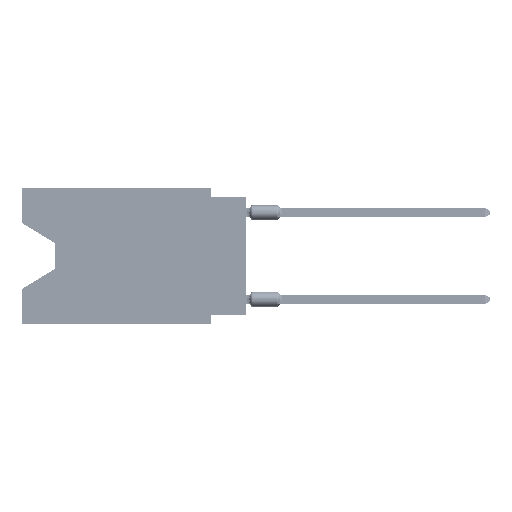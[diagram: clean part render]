
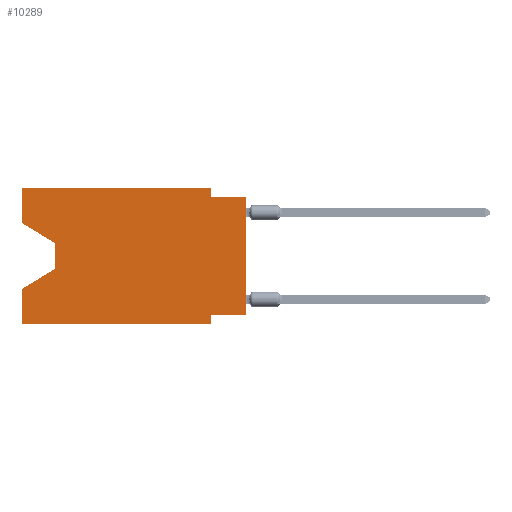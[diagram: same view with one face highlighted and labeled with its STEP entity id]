
A CAD part, left-side view. The second image highlights one B-rep face of the part: STEP entity #10289.
In plain terms, the highlighted planar face has unit normal (-1, 0, 0).
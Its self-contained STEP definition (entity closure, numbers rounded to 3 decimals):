
#3609 = DIRECTION ( 'NONE',  ( 0., 0., 1. ) ) ;
#4931 = EDGE_CURVE ( 'NONE', #17373, #41994, #17701, .T. ) ;
#6019 = FACE_OUTER_BOUND ( 'NONE', #15911, .T. ) ;
#6279 = CARTESIAN_POINT ( 'NONE',  ( 0., 16.383, -2.546 ) ) ;
#6322 = DIRECTION ( 'NONE',  ( 0., 0., -1. ) ) ;
#7239 = VERTEX_POINT ( 'NONE', #69543 ) ;
#7958 = VERTEX_POINT ( 'NONE', #50882 ) ;
#7977 = ORIENTED_EDGE ( 'NONE', *, *, #4931, .F. ) ;
#9017 = EDGE_CURVE ( 'NONE', #26967, #64540, #48425, .T. ) ;
#9686 = LINE ( 'NONE', #20018, #24121 ) ;
#10289 = ADVANCED_FACE ( 'NONE', ( #6019 ), #59487, .F. ) ;
#10655 = DIRECTION ( 'NONE',  ( 0., 0., -1. ) ) ;
#13423 = CARTESIAN_POINT ( 'NONE',  ( 0., 13.97, -4.013 ) ) ;
#13834 = DIRECTION ( 'NONE',  ( 0., 0., -1. ) ) ;
#14035 = VECTOR ( 'NONE', #3609, 1000. ) ;
#14691 = DIRECTION ( 'NONE',  ( 0., 0., 1. ) ) ;
#15911 = EDGE_LOOP ( 'NONE', ( #19142, #49990, #54286, #69501, #42773, #57757, #22261, #31472, #7977, #49883, #57065, #53916 ) ) ;
#16721 = EDGE_CURVE ( 'NONE', #33170, #17373, #61953, .T. ) ;
#17373 = VERTEX_POINT ( 'NONE', #43285 ) ;
#17701 = LINE ( 'NONE', #24094, #46990 ) ;
#19111 = LINE ( 'NONE', #13423, #55310 ) ;
#19142 = ORIENTED_EDGE ( 'NONE', *, *, #69647, .T. ) ;
#19218 = VERTEX_POINT ( 'NONE', #56373 ) ;
#19702 = DIRECTION ( 'NONE',  ( 0., -0.855, -0.519 ) ) ;
#20018 = CARTESIAN_POINT ( 'NONE',  ( 0., 16.383, 0. ) ) ;
#21085 = DIRECTION ( 'NONE',  ( 0., 1., 0. ) ) ;
#21438 = CARTESIAN_POINT ( 'NONE',  ( 0., 0., -9.271 ) ) ;
#22261 = ORIENTED_EDGE ( 'NONE', *, *, #41687, .F. ) ;
#22366 = CARTESIAN_POINT ( 'NONE',  ( 0., 2.54, -9.906 ) ) ;
#22782 = VECTOR ( 'NONE', #19702, 1000. ) ;
#23371 = EDGE_CURVE ( 'NONE', #54502, #41994, #64180, .T. ) ;
#23584 = CARTESIAN_POINT ( 'NONE',  ( 0., 13.97, -5.893 ) ) ;
#24094 = CARTESIAN_POINT ( 'NONE',  ( 0., 0., -0.635 ) ) ;
#24121 = VECTOR ( 'NONE', #14691, 1000. ) ;
#24172 = DIRECTION ( 'NONE',  ( 0., 0., 1. ) ) ;
#24516 = CARTESIAN_POINT ( 'NONE',  ( 0., 16.383, 0. ) ) ;
#26543 = DIRECTION ( 'NONE',  ( 0., 0.855, -0.519 ) ) ;
#26967 = VERTEX_POINT ( 'NONE', #42232 ) ;
#27241 = CARTESIAN_POINT ( 'NONE',  ( 0., 13.97, -5.893 ) ) ;
#27286 = VECTOR ( 'NONE', #26543, 1000. ) ;
#27478 = CARTESIAN_POINT ( 'NONE',  ( 0., 2.54, -9.906 ) ) ;
#27803 = EDGE_CURVE ( 'NONE', #26967, #7239, #50575, .T. ) ;
#28559 = VERTEX_POINT ( 'NONE', #65169 ) ;
#29102 = VECTOR ( 'NONE', #63996, 1000. ) ;
#31472 = ORIENTED_EDGE ( 'NONE', *, *, #23371, .T. ) ;
#31867 = VECTOR ( 'NONE', #24172, 1000. ) ;
#33170 = VERTEX_POINT ( 'NONE', #60333 ) ;
#34088 = LINE ( 'NONE', #6279, #22782 ) ;
#35867 = DIRECTION ( 'NONE',  ( 0., 0., -1. ) ) ;
#36252 = EDGE_CURVE ( 'NONE', #19218, #33170, #41887, .T. ) ;
#37494 = LINE ( 'NONE', #21438, #50350 ) ;
#38062 = VERTEX_POINT ( 'NONE', #23584 ) ;
#38452 = CARTESIAN_POINT ( 'NONE',  ( 0., 16.383, 0. ) ) ;
#38802 = DIRECTION ( 'NONE',  ( 0., -1., 0. ) ) ;
#39440 = DIRECTION ( 'NONE',  ( 0., -1., 0. ) ) ;
#41346 = EDGE_CURVE ( 'NONE', #38062, #7239, #42912, .T. ) ;
#41687 = EDGE_CURVE ( 'NONE', #54502, #28559, #37494, .T. ) ;
#41887 = LINE ( 'NONE', #62925, #29102 ) ;
#41994 = VERTEX_POINT ( 'NONE', #45434 ) ;
#42232 = CARTESIAN_POINT ( 'NONE',  ( 0., 16.383, -9.906 ) ) ;
#42654 = EDGE_CURVE ( 'NONE', #7958, #19218, #9686, .T. ) ;
#42773 = ORIENTED_EDGE ( 'NONE', *, *, #9017, .T. ) ;
#42912 = LINE ( 'NONE', #27241, #27286 ) ;
#43273 = VECTOR ( 'NONE', #6322, 1000. ) ;
#43285 = CARTESIAN_POINT ( 'NONE',  ( 0., 2.54, -0.635 ) ) ;
#43766 = CARTESIAN_POINT ( 'NONE',  ( 0., 16.383, -9.906 ) ) ;
#45434 = CARTESIAN_POINT ( 'NONE',  ( 0., 0., -0.635 ) ) ;
#46362 = VECTOR ( 'NONE', #13834, 1000. ) ;
#46990 = VECTOR ( 'NONE', #39440, 1000. ) ;
#47098 = CARTESIAN_POINT ( 'NONE',  ( 0., 0., -9.271 ) ) ;
#48056 = CARTESIAN_POINT ( 'NONE',  ( 0., 13.97, -4.013 ) ) ;
#48425 = LINE ( 'NONE', #43766, #51933 ) ;
#49500 = DIRECTION ( 'NONE',  ( 1., 0., 0. ) ) ;
#49883 = ORIENTED_EDGE ( 'NONE', *, *, #16721, .F. ) ;
#49990 = ORIENTED_EDGE ( 'NONE', *, *, #62215, .T. ) ;
#50350 = VECTOR ( 'NONE', #21085, 1000. ) ;
#50575 = LINE ( 'NONE', #24516, #31867 ) ;
#50882 = CARTESIAN_POINT ( 'NONE',  ( 0., 16.383, -2.546 ) ) ;
#51933 = VECTOR ( 'NONE', #38802, 1000. ) ;
#52252 = VERTEX_POINT ( 'NONE', #48056 ) ;
#53916 = ORIENTED_EDGE ( 'NONE', *, *, #42654, .F. ) ;
#54286 = ORIENTED_EDGE ( 'NONE', *, *, #41346, .T. ) ;
#54455 = LINE ( 'NONE', #22366, #43273 ) ;
#54502 = VERTEX_POINT ( 'NONE', #47098 ) ;
#55310 = VECTOR ( 'NONE', #35867, 1000. ) ;
#56373 = CARTESIAN_POINT ( 'NONE',  ( 0., 16.383, 0. ) ) ;
#56953 = CARTESIAN_POINT ( 'NONE',  ( 0., 2.54, 0. ) ) ;
#57065 = ORIENTED_EDGE ( 'NONE', *, *, #36252, .F. ) ;
#57561 = AXIS2_PLACEMENT_3D ( 'NONE', #38452, #49500, #10655 ) ;
#57757 = ORIENTED_EDGE ( 'NONE', *, *, #69452, .F. ) ;
#59487 = PLANE ( 'NONE',  #57561 ) ;
#60333 = CARTESIAN_POINT ( 'NONE',  ( 0., 2.54, 0. ) ) ;
#61953 = LINE ( 'NONE', #56953, #46362 ) ;
#62215 = EDGE_CURVE ( 'NONE', #52252, #38062, #19111, .T. ) ;
#62925 = CARTESIAN_POINT ( 'NONE',  ( 0., 16.383, 0. ) ) ;
#63484 = CARTESIAN_POINT ( 'NONE',  ( 0., 0., 0. ) ) ;
#63996 = DIRECTION ( 'NONE',  ( 0., -1., 0. ) ) ;
#64180 = LINE ( 'NONE', #63484, #14035 ) ;
#64540 = VERTEX_POINT ( 'NONE', #27478 ) ;
#65169 = CARTESIAN_POINT ( 'NONE',  ( 0., 2.54, -9.271 ) ) ;
#69452 = EDGE_CURVE ( 'NONE', #28559, #64540, #54455, .T. ) ;
#69501 = ORIENTED_EDGE ( 'NONE', *, *, #27803, .F. ) ;
#69543 = CARTESIAN_POINT ( 'NONE',  ( 0., 16.383, -7.36 ) ) ;
#69647 = EDGE_CURVE ( 'NONE', #7958, #52252, #34088, .T. ) ;
